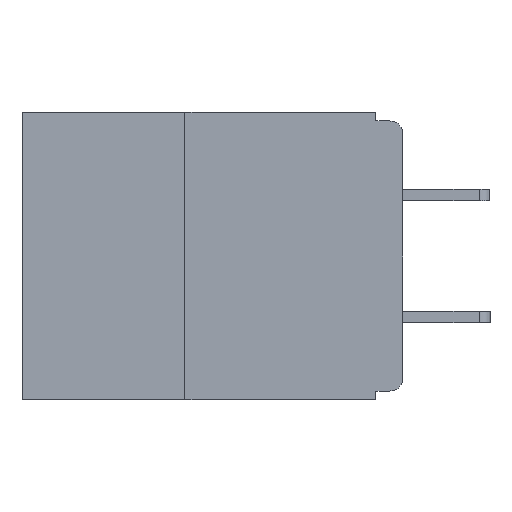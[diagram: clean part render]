
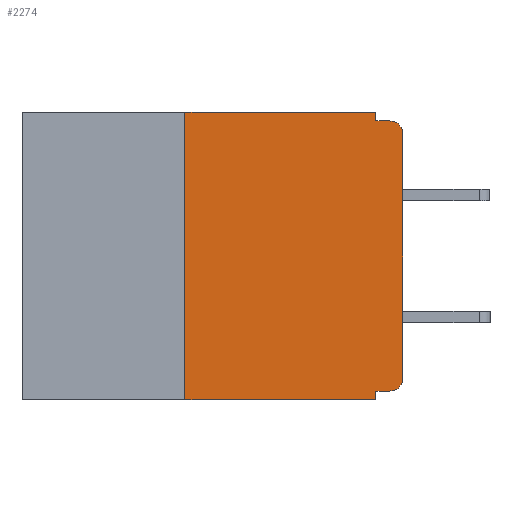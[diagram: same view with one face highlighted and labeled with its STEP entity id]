
A CAD part, left-side view. The second image highlights one B-rep face of the part: STEP entity #2274.
In plain terms, the highlighted planar face has unit normal (-1, 0, 0).
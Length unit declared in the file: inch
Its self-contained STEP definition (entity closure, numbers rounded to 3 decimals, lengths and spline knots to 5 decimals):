
#14 = DIRECTION ( 'NONE',  ( 0., -1., 0. ) ) ;
#124 = CARTESIAN_POINT ( 'NONE',  ( 0., 0.25, 0. ) ) ;
#160 = AXIS2_PLACEMENT_3D ( 'NONE', #6534, #6187, #8487 ) ;
#777 = EDGE_CURVE ( 'NONE', #8475, #14101, #16949, .T. ) ;
#1138 = AXIS2_PLACEMENT_3D ( 'NONE', #10604, #2306, #8255 ) ;
#1143 = CARTESIAN_POINT ( 'NONE',  ( 0., 0., -0.025 ) ) ;
#1674 = VERTEX_POINT ( 'NONE', #7758 ) ;
#2274 = ADVANCED_FACE ( 'NONE', ( #9290 ), #5703, .F. ) ;
#2306 = DIRECTION ( 'NONE',  ( 1., 0., 0. ) ) ;
#2386 = EDGE_CURVE ( 'NONE', #13580, #1674, #10781, .T. ) ;
#2924 = VERTEX_POINT ( 'NONE', #5241 ) ;
#3295 = CARTESIAN_POINT ( 'NONE',  ( 0., 0.015, -0.01 ) ) ;
#3678 = CARTESIAN_POINT ( 'NONE',  ( 0., 0.031, -0.33 ) ) ;
#3736 = CIRCLE ( 'NONE', #10154, 0.015 ) ;
#4254 = LINE ( 'NONE', #13895, #11018 ) ;
#4267 = LINE ( 'NONE', #10065, #6012 ) ;
#4395 = LINE ( 'NONE', #7146, #5242 ) ;
#4470 = VERTEX_POINT ( 'NONE', #6385 ) ;
#4755 = CARTESIAN_POINT ( 'NONE',  ( 0., 0.031, 0. ) ) ;
#5241 = CARTESIAN_POINT ( 'NONE',  ( 0., 0., -0.305 ) ) ;
#5242 = VECTOR ( 'NONE', #8497, 39.37008 ) ;
#5351 = EDGE_CURVE ( 'NONE', #12065, #2924, #3736, .T. ) ;
#5456 = EDGE_CURVE ( 'NONE', #2924, #8475, #12816, .T. ) ;
#5459 = EDGE_CURVE ( 'NONE', #12065, #13580, #5711, .T. ) ;
#5703 = PLANE ( 'NONE',  #1138 ) ;
#5711 = LINE ( 'NONE', #6717, #15894 ) ;
#6012 = VECTOR ( 'NONE', #12753, 39.37008 ) ;
#6187 = DIRECTION ( 'NONE',  ( -1., 0., 0. ) ) ;
#6241 = DIRECTION ( 'NONE',  ( 0., 1., 0. ) ) ;
#6385 = CARTESIAN_POINT ( 'NONE',  ( 0., 0.031, -0.01 ) ) ;
#6534 = CARTESIAN_POINT ( 'NONE',  ( 0., 0.015, -0.025 ) ) ;
#6717 = CARTESIAN_POINT ( 'NONE',  ( 0., 0., -0.32 ) ) ;
#6950 = DIRECTION ( 'NONE',  ( 0., 0., 1. ) ) ;
#6974 = CARTESIAN_POINT ( 'NONE',  ( 0., 0.437, 0. ) ) ;
#7146 = CARTESIAN_POINT ( 'NONE',  ( 0., 0.25, -0.33 ) ) ;
#7221 = DIRECTION ( 'NONE',  ( 0., 0., -1. ) ) ;
#7243 = LINE ( 'NONE', #6974, #10841 ) ;
#7541 = CARTESIAN_POINT ( 'NONE',  ( 0., 0., 0. ) ) ;
#7758 = CARTESIAN_POINT ( 'NONE',  ( 0., 0.031, -0.33 ) ) ;
#7911 = EDGE_CURVE ( 'NONE', #8543, #1674, #8325, .T. ) ;
#8255 = DIRECTION ( 'NONE',  ( 0., 0., -1. ) ) ;
#8325 = LINE ( 'NONE', #15004, #11515 ) ;
#8475 = VERTEX_POINT ( 'NONE', #1143 ) ;
#8487 = DIRECTION ( 'NONE',  ( 0., 0., -1. ) ) ;
#8497 = DIRECTION ( 'NONE',  ( 0., 0., 1. ) ) ;
#8543 = VERTEX_POINT ( 'NONE', #12487 ) ;
#9172 = EDGE_CURVE ( 'NONE', #13209, #10983, #7243, .T. ) ;
#9290 = FACE_OUTER_BOUND ( 'NONE', #13404, .T. ) ;
#9822 = DIRECTION ( 'NONE',  ( 0., 0., -1. ) ) ;
#9858 = DIRECTION ( 'NONE',  ( -1., 0., 0. ) ) ;
#10065 = CARTESIAN_POINT ( 'NONE',  ( 0., 0., -0.01 ) ) ;
#10101 = VECTOR ( 'NONE', #6950, 39.37008 ) ;
#10154 = AXIS2_PLACEMENT_3D ( 'NONE', #10247, #9858, #9822 ) ;
#10247 = CARTESIAN_POINT ( 'NONE',  ( 0., 0.015, -0.305 ) ) ;
#10604 = CARTESIAN_POINT ( 'NONE',  ( 0., 0.437, 0. ) ) ;
#10781 = LINE ( 'NONE', #3678, #17276 ) ;
#10841 = VECTOR ( 'NONE', #14, 39.37008 ) ;
#10983 = VERTEX_POINT ( 'NONE', #4755 ) ;
#11018 = VECTOR ( 'NONE', #7221, 39.37008 ) ;
#11515 = VECTOR ( 'NONE', #16221, 39.37008 ) ;
#11540 = EDGE_CURVE ( 'NONE', #8543, #13209, #4395, .T. ) ;
#12065 = VERTEX_POINT ( 'NONE', #13439 ) ;
#12487 = CARTESIAN_POINT ( 'NONE',  ( 0., 0.25, -0.33 ) ) ;
#12753 = DIRECTION ( 'NONE',  ( 0., -1., 0. ) ) ;
#12816 = LINE ( 'NONE', #7541, #10101 ) ;
#13192 = ORIENTED_EDGE ( 'NONE', *, *, #5456, .T. ) ;
#13209 = VERTEX_POINT ( 'NONE', #124 ) ;
#13303 = ORIENTED_EDGE ( 'NONE', *, *, #777, .T. ) ;
#13350 = ORIENTED_EDGE ( 'NONE', *, *, #17031, .F. ) ;
#13404 = EDGE_LOOP ( 'NONE', ( #13192, #13303, #13350, #13511, #13540, #13663, #13916, #14094, #14127, #14956 ) ) ;
#13439 = CARTESIAN_POINT ( 'NONE',  ( 0., 0.015, -0.32 ) ) ;
#13511 = ORIENTED_EDGE ( 'NONE', *, *, #15923, .F. ) ;
#13540 = ORIENTED_EDGE ( 'NONE', *, *, #9172, .F. ) ;
#13580 = VERTEX_POINT ( 'NONE', #16971 ) ;
#13663 = ORIENTED_EDGE ( 'NONE', *, *, #11540, .F. ) ;
#13819 = DIRECTION ( 'NONE',  ( 0., 0., -1. ) ) ;
#13895 = CARTESIAN_POINT ( 'NONE',  ( 0., 0.031, 0. ) ) ;
#13916 = ORIENTED_EDGE ( 'NONE', *, *, #7911, .T. ) ;
#14094 = ORIENTED_EDGE ( 'NONE', *, *, #2386, .F. ) ;
#14101 = VERTEX_POINT ( 'NONE', #3295 ) ;
#14127 = ORIENTED_EDGE ( 'NONE', *, *, #5459, .F. ) ;
#14956 = ORIENTED_EDGE ( 'NONE', *, *, #5351, .T. ) ;
#15004 = CARTESIAN_POINT ( 'NONE',  ( 0., 0.437, -0.33 ) ) ;
#15894 = VECTOR ( 'NONE', #6241, 39.37008 ) ;
#15923 = EDGE_CURVE ( 'NONE', #10983, #4470, #4254, .T. ) ;
#16221 = DIRECTION ( 'NONE',  ( 0., -1., 0. ) ) ;
#16949 = CIRCLE ( 'NONE', #160, 0.015 ) ;
#16971 = CARTESIAN_POINT ( 'NONE',  ( 0., 0.031, -0.32 ) ) ;
#17031 = EDGE_CURVE ( 'NONE', #4470, #14101, #4267, .T. ) ;
#17276 = VECTOR ( 'NONE', #13819, 39.37008 ) ;
